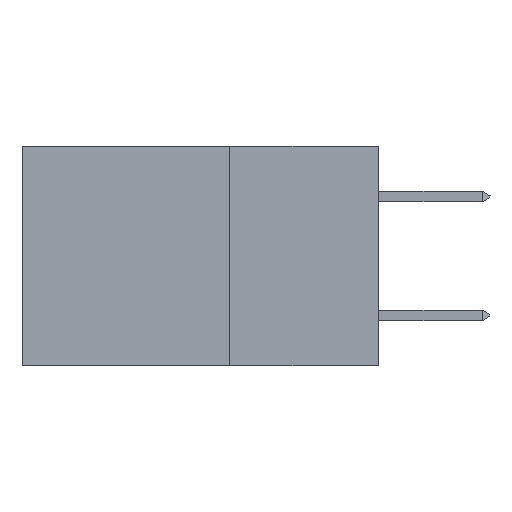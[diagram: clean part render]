
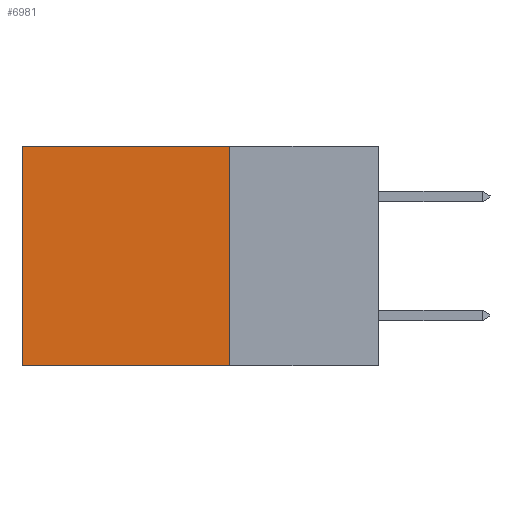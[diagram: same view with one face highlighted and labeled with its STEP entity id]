
A CAD part, left-side view. The second image highlights one B-rep face of the part: STEP entity #6981.
In plain terms, the highlighted planar face has unit normal (-1, 0, 0).
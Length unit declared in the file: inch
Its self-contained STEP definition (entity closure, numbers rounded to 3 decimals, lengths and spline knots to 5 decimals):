
#246 = CARTESIAN_POINT ( 'NONE',  ( 0.2615, 0.25, -0.37 ) ) ;
#447 = ORIENTED_EDGE ( 'NONE', *, *, #8862, .F. ) ;
#554 = PLANE ( 'NONE',  #3831 ) ;
#1620 = CARTESIAN_POINT ( 'NONE',  ( 0.2615, 0.25, -0.37 ) ) ;
#1823 = ORIENTED_EDGE ( 'NONE', *, *, #12006, .T. ) ;
#2448 = CARTESIAN_POINT ( 'NONE',  ( 0.2615, 0.6, -0.37 ) ) ;
#3674 = LINE ( 'NONE', #25610, #7763 ) ;
#3831 = AXIS2_PLACEMENT_3D ( 'NONE', #8462, #14914, #18939 ) ;
#3851 = DIRECTION ( 'NONE',  ( 0., 1., 0. ) ) ;
#3972 = LINE ( 'NONE', #1620, #15954 ) ;
#4610 = VERTEX_POINT ( 'NONE', #8775 ) ;
#5531 = VECTOR ( 'NONE', #20095, 39.37008 ) ;
#6360 = CARTESIAN_POINT ( 'NONE',  ( 0.2615, 0.6, 0. ) ) ;
#6479 = LINE ( 'NONE', #2448, #8897 ) ;
#6981 = ADVANCED_FACE ( 'NONE', ( #18323 ), #554, .F. ) ;
#7763 = VECTOR ( 'NONE', #11580, 39.37008 ) ;
#8288 = LINE ( 'NONE', #246, #5531 ) ;
#8462 = CARTESIAN_POINT ( 'NONE',  ( 0.2615, 0.25, -0.37 ) ) ;
#8775 = CARTESIAN_POINT ( 'NONE',  ( 0.2615, 0.25, 0. ) ) ;
#8802 = VERTEX_POINT ( 'NONE', #6360 ) ;
#8862 = EDGE_CURVE ( 'NONE', #4610, #12157, #8288, .T. ) ;
#8897 = VECTOR ( 'NONE', #16811, 39.37008 ) ;
#10113 = CARTESIAN_POINT ( 'NONE',  ( 0.2615, 0.6, -0.37 ) ) ;
#11580 = DIRECTION ( 'NONE',  ( 0., 1., 0. ) ) ;
#12006 = EDGE_CURVE ( 'NONE', #8802, #17143, #6479, .T. ) ;
#12157 = VERTEX_POINT ( 'NONE', #20847 ) ;
#12384 = ORIENTED_EDGE ( 'NONE', *, *, #20961, .T. ) ;
#12863 = EDGE_CURVE ( 'NONE', #12157, #17143, #3972, .T. ) ;
#14914 = DIRECTION ( 'NONE',  ( 1., 0., 0. ) ) ;
#15954 = VECTOR ( 'NONE', #3851, 39.37008 ) ;
#16162 = ORIENTED_EDGE ( 'NONE', *, *, #12863, .F. ) ;
#16811 = DIRECTION ( 'NONE',  ( 0., 0., -1. ) ) ;
#17143 = VERTEX_POINT ( 'NONE', #10113 ) ;
#18323 = FACE_OUTER_BOUND ( 'NONE', #24357, .T. ) ;
#18939 = DIRECTION ( 'NONE',  ( 0., 0., -1. ) ) ;
#20095 = DIRECTION ( 'NONE',  ( 0., 0., -1. ) ) ;
#20847 = CARTESIAN_POINT ( 'NONE',  ( 0.2615, 0.25, -0.37 ) ) ;
#20961 = EDGE_CURVE ( 'NONE', #4610, #8802, #3674, .T. ) ;
#24357 = EDGE_LOOP ( 'NONE', ( #1823, #16162, #447, #12384 ) ) ;
#25610 = CARTESIAN_POINT ( 'NONE',  ( 0.2615, 0.25, 0. ) ) ;
